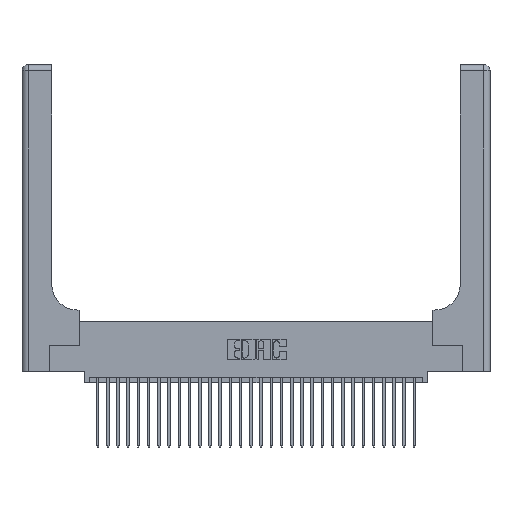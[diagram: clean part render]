
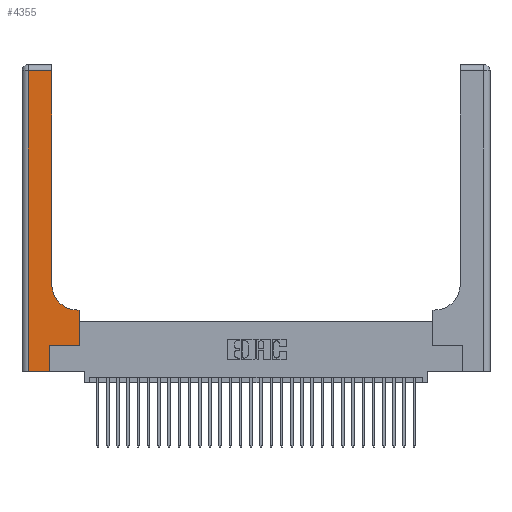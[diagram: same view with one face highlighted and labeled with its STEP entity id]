
A CAD part, top view. The second image highlights one B-rep face of the part: STEP entity #4355.
In plain terms, the highlighted planar face has unit normal (0, 0, 1).
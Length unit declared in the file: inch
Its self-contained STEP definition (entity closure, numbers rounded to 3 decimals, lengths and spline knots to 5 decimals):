
#50 = PLANE ( 'NONE',  #18989 ) ;
#584 = VERTEX_POINT ( 'NONE', #28327 ) ;
#1262 = VERTEX_POINT ( 'NONE', #6814 ) ;
#1359 = EDGE_CURVE ( 'NONE', #19804, #9242, #3169, .T. ) ;
#1544 = DIRECTION ( 'NONE',  ( -1., 0., 0. ) ) ;
#1772 = DIRECTION ( 'NONE',  ( 0., 0., -1. ) ) ;
#2257 = ORIENTED_EDGE ( 'NONE', *, *, #8036, .T. ) ;
#2345 = EDGE_CURVE ( 'NONE', #10322, #10384, #25797, .T. ) ;
#3155 = ORIENTED_EDGE ( 'NONE', *, *, #10144, .T. ) ;
#3159 = DIRECTION ( 'NONE',  ( -1., 0., 0. ) ) ;
#3169 = LINE ( 'NONE', #10217, #18629 ) ;
#3233 = EDGE_LOOP ( 'NONE', ( #11189, #8897, #7938, #3155, #14787, #21835, #27887, #2257, #9706 ) ) ;
#4142 = DIRECTION ( 'NONE',  ( -1., 0., 0. ) ) ;
#4236 = VERTEX_POINT ( 'NONE', #13553 ) ;
#4355 = ADVANCED_FACE ( 'NONE', ( #13804 ), #50, .F. ) ;
#6265 = CARTESIAN_POINT ( 'NONE',  ( 0.5415, 0.6, 0.37 ) ) ;
#6526 = CARTESIAN_POINT ( 'NONE',  ( 0., 3., 0.37 ) ) ;
#6814 = CARTESIAN_POINT ( 'NONE',  ( 0.2915, 2.94, 0.37 ) ) ;
#7517 = CARTESIAN_POINT ( 'NONE',  ( 0.5585, 0.6, 0.37 ) ) ;
#7892 = LINE ( 'NONE', #18768, #27506 ) ;
#7938 = ORIENTED_EDGE ( 'NONE', *, *, #25163, .T. ) ;
#8036 = EDGE_CURVE ( 'NONE', #9242, #10322, #19803, .T. ) ;
#8443 = CARTESIAN_POINT ( 'NONE',  ( 0.269, 0., 0.37 ) ) ;
#8882 = CARTESIAN_POINT ( 'NONE',  ( 0., 2.94, 0.37 ) ) ;
#8897 = ORIENTED_EDGE ( 'NONE', *, *, #20070, .T. ) ;
#9242 = VERTEX_POINT ( 'NONE', #7517 ) ;
#9706 = ORIENTED_EDGE ( 'NONE', *, *, #2345, .T. ) ;
#10144 = EDGE_CURVE ( 'NONE', #584, #20523, #28487, .T. ) ;
#10217 = CARTESIAN_POINT ( 'NONE',  ( 0.5585, 0.25, 0.37 ) ) ;
#10322 = VERTEX_POINT ( 'NONE', #6265 ) ;
#10384 = VERTEX_POINT ( 'NONE', #29429 ) ;
#10397 = CARTESIAN_POINT ( 'NONE',  ( 0.5585, 0.25, 0.37 ) ) ;
#11189 = ORIENTED_EDGE ( 'NONE', *, *, #22278, .T. ) ;
#11791 = LINE ( 'NONE', #13237, #17622 ) ;
#12791 = CARTESIAN_POINT ( 'NONE',  ( 0.5415, 0.85, 0.37 ) ) ;
#13193 = VECTOR ( 'NONE', #31635, 39.37008 ) ;
#13237 = CARTESIAN_POINT ( 'NONE',  ( 0.2915, 3., 0.37 ) ) ;
#13553 = CARTESIAN_POINT ( 'NONE',  ( 0.269, 0.25, 0.37 ) ) ;
#13804 = FACE_OUTER_BOUND ( 'NONE', #3233, .T. ) ;
#14787 = ORIENTED_EDGE ( 'NONE', *, *, #21819, .T. ) ;
#14934 = DIRECTION ( 'NONE',  ( 1., 0., 0. ) ) ;
#15302 = DIRECTION ( 'NONE',  ( 1., 0., 0. ) ) ;
#17137 = VECTOR ( 'NONE', #3159, 39.37008 ) ;
#17622 = VECTOR ( 'NONE', #28303, 39.37008 ) ;
#17733 = AXIS2_PLACEMENT_3D ( 'NONE', #12791, #29915, #15302 ) ;
#17954 = CARTESIAN_POINT ( 'NONE',  ( 0.2915, 0.6, 0.37 ) ) ;
#18629 = VECTOR ( 'NONE', #27382, 39.37008 ) ;
#18768 = CARTESIAN_POINT ( 'NONE',  ( 0.269, 0.25, 0.37 ) ) ;
#18989 = AXIS2_PLACEMENT_3D ( 'NONE', #6526, #1772, #4142 ) ;
#19803 = LINE ( 'NONE', #17954, #17137 ) ;
#19804 = VERTEX_POINT ( 'NONE', #10397 ) ;
#19944 = VECTOR ( 'NONE', #28661, 39.37008 ) ;
#20070 = EDGE_CURVE ( 'NONE', #1262, #23516, #22654, .T. ) ;
#20329 = LINE ( 'NONE', #28348, #19944 ) ;
#20523 = VERTEX_POINT ( 'NONE', #8443 ) ;
#21819 = EDGE_CURVE ( 'NONE', #20523, #4236, #20329, .T. ) ;
#21835 = ORIENTED_EDGE ( 'NONE', *, *, #28685, .T. ) ;
#22278 = EDGE_CURVE ( 'NONE', #10384, #1262, #11791, .T. ) ;
#22654 = LINE ( 'NONE', #8882, #26099 ) ;
#23139 = LINE ( 'NONE', #29059, #13193 ) ;
#23516 = VERTEX_POINT ( 'NONE', #27654 ) ;
#25163 = EDGE_CURVE ( 'NONE', #23516, #584, #23139, .T. ) ;
#25797 = CIRCLE ( 'NONE', #17733, 0.25 ) ;
#26099 = VECTOR ( 'NONE', #1544, 39.37008 ) ;
#26112 = DIRECTION ( 'NONE',  ( 1., 0., 0. ) ) ;
#27382 = DIRECTION ( 'NONE',  ( 0., 1., 0. ) ) ;
#27506 = VECTOR ( 'NONE', #26112, 39.37008 ) ;
#27654 = CARTESIAN_POINT ( 'NONE',  ( 0.06, 2.94, 0.37 ) ) ;
#27887 = ORIENTED_EDGE ( 'NONE', *, *, #1359, .T. ) ;
#28303 = DIRECTION ( 'NONE',  ( 0., 1., 0. ) ) ;
#28327 = CARTESIAN_POINT ( 'NONE',  ( 0.06, 0., 0.37 ) ) ;
#28348 = CARTESIAN_POINT ( 'NONE',  ( 0.269, 0., 0.37 ) ) ;
#28487 = LINE ( 'NONE', #29558, #30385 ) ;
#28661 = DIRECTION ( 'NONE',  ( 0., 1., 0. ) ) ;
#28685 = EDGE_CURVE ( 'NONE', #4236, #19804, #7892, .T. ) ;
#29059 = CARTESIAN_POINT ( 'NONE',  ( 0.06, 3., 0.37 ) ) ;
#29429 = CARTESIAN_POINT ( 'NONE',  ( 0.2915, 0.85, 0.37 ) ) ;
#29558 = CARTESIAN_POINT ( 'NONE',  ( 0., 0., 0.37 ) ) ;
#29915 = DIRECTION ( 'NONE',  ( 0., 0., -1. ) ) ;
#30385 = VECTOR ( 'NONE', #14934, 39.37008 ) ;
#31635 = DIRECTION ( 'NONE',  ( 0., -1., 0. ) ) ;
